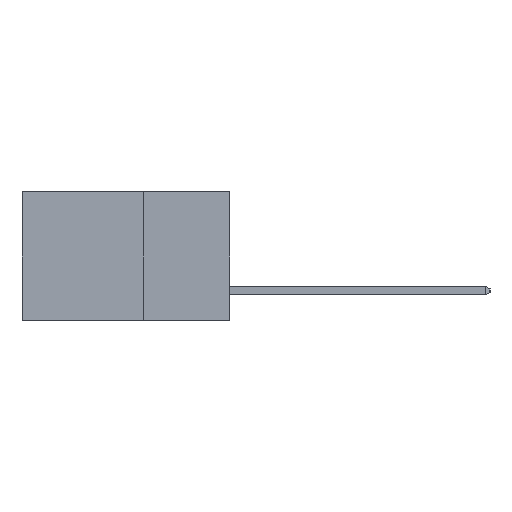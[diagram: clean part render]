
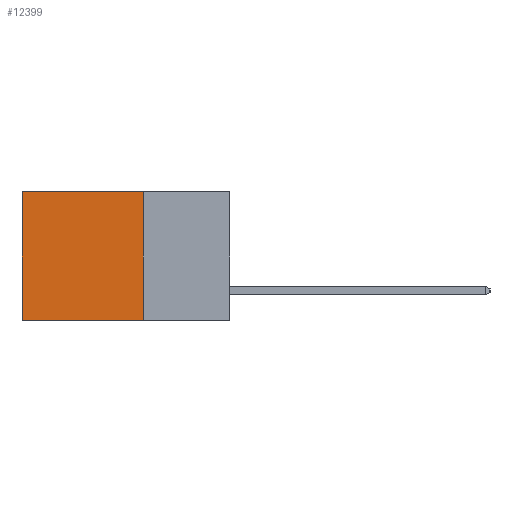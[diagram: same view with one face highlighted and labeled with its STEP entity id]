
A CAD part, left-side view. The second image highlights one B-rep face of the part: STEP entity #12399.
In plain terms, the highlighted planar face has unit normal (-1, 0, 0).
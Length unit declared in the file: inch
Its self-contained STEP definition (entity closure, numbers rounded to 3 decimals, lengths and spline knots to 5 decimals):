
#876 = EDGE_LOOP ( 'NONE', ( #2440, #1470, #5463, #14930 ) ) ;
#1470 = ORIENTED_EDGE ( 'NONE', *, *, #4888, .F. ) ;
#1772 = VECTOR ( 'NONE', #15187, 39.37008 ) ;
#2300 = LINE ( 'NONE', #7258, #9987 ) ;
#2440 = ORIENTED_EDGE ( 'NONE', *, *, #13010, .T. ) ;
#2966 = CARTESIAN_POINT ( 'NONE',  ( 0.2615, 0.6, -0.37 ) ) ;
#4485 = CARTESIAN_POINT ( 'NONE',  ( 0.2615, 0.25, -0.37 ) ) ;
#4888 = EDGE_CURVE ( 'NONE', #14681, #16105, #2300, .T. ) ;
#5257 = VECTOR ( 'NONE', #8909, 39.37008 ) ;
#5463 = ORIENTED_EDGE ( 'NONE', *, *, #12272, .F. ) ;
#5734 = LINE ( 'NONE', #7314, #5257 ) ;
#6706 = LINE ( 'NONE', #15403, #18226 ) ;
#7258 = CARTESIAN_POINT ( 'NONE',  ( 0.2615, 0.25, -0.37 ) ) ;
#7314 = CARTESIAN_POINT ( 'NONE',  ( 0.2615, 0.25, -0.37 ) ) ;
#7637 = DIRECTION ( 'NONE',  ( 1., 0., 0. ) ) ;
#8909 = DIRECTION ( 'NONE',  ( 0., 0., -1. ) ) ;
#9987 = VECTOR ( 'NONE', #18100, 39.37008 ) ;
#10151 = VERTEX_POINT ( 'NONE', #12513 ) ;
#12272 = EDGE_CURVE ( 'NONE', #10151, #14681, #5734, .T. ) ;
#12399 = ADVANCED_FACE ( 'NONE', ( #18890 ), #13716, .F. ) ;
#12513 = CARTESIAN_POINT ( 'NONE',  ( 0.2615, 0.25, 0. ) ) ;
#13010 = EDGE_CURVE ( 'NONE', #18304, #16105, #17912, .T. ) ;
#13258 = CARTESIAN_POINT ( 'NONE',  ( 0.2615, 0.25, -0.37 ) ) ;
#13716 = PLANE ( 'NONE',  #18250 ) ;
#14681 = VERTEX_POINT ( 'NONE', #13258 ) ;
#14930 = ORIENTED_EDGE ( 'NONE', *, *, #16858, .T. ) ;
#15187 = DIRECTION ( 'NONE',  ( 0., 0., -1. ) ) ;
#15403 = CARTESIAN_POINT ( 'NONE',  ( 0.2615, 0.25, 0. ) ) ;
#16105 = VERTEX_POINT ( 'NONE', #19537 ) ;
#16540 = CARTESIAN_POINT ( 'NONE',  ( 0.2615, 0.6, 0. ) ) ;
#16858 = EDGE_CURVE ( 'NONE', #10151, #18304, #6706, .T. ) ;
#16880 = DIRECTION ( 'NONE',  ( 0., 1., 0. ) ) ;
#17912 = LINE ( 'NONE', #2966, #1772 ) ;
#18100 = DIRECTION ( 'NONE',  ( 0., 1., 0. ) ) ;
#18149 = DIRECTION ( 'NONE',  ( 0., 0., -1. ) ) ;
#18226 = VECTOR ( 'NONE', #16880, 39.37008 ) ;
#18250 = AXIS2_PLACEMENT_3D ( 'NONE', #4485, #7637, #18149 ) ;
#18304 = VERTEX_POINT ( 'NONE', #16540 ) ;
#18890 = FACE_OUTER_BOUND ( 'NONE', #876, .T. ) ;
#19537 = CARTESIAN_POINT ( 'NONE',  ( 0.2615, 0.6, -0.37 ) ) ;
